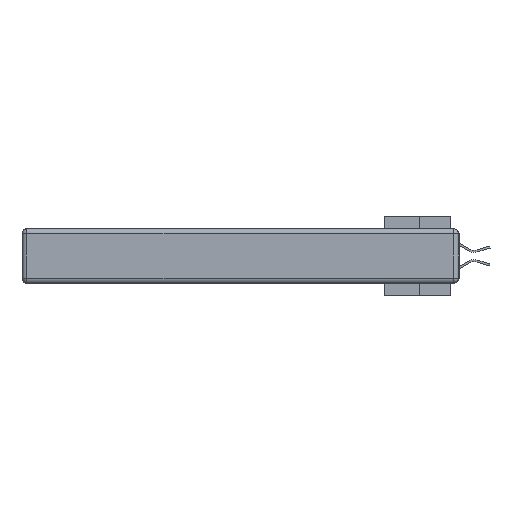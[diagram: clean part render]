
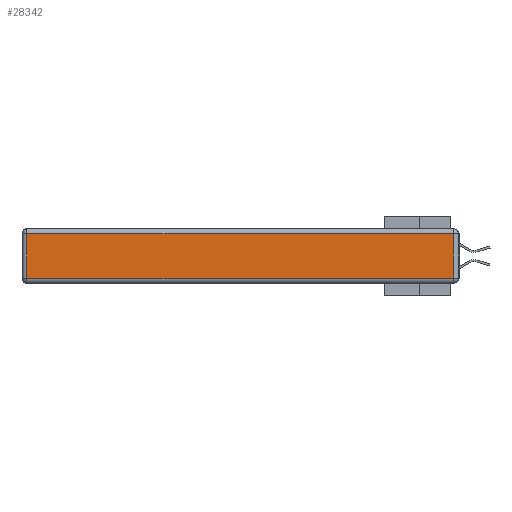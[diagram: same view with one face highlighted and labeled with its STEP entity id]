
A CAD part, left-side view. The second image highlights one B-rep face of the part: STEP entity #28342.
In plain terms, the highlighted planar face has unit normal (-1, 0, 0).
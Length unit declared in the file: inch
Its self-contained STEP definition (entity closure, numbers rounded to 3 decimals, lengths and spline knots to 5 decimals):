
#481 = CARTESIAN_POINT ( 'NONE',  ( 0., 0., -0.343 ) ) ;
#520 = CARTESIAN_POINT ( 'NONE',  ( 0., 0.03, -0.313 ) ) ;
#1318 = DIRECTION ( 'NONE',  ( 0., -1., 0. ) ) ;
#1412 = EDGE_CURVE ( 'NONE', #2188, #10132, #20508, .T. ) ;
#1446 = DIRECTION ( 'NONE',  ( 0., 0., -1. ) ) ;
#2188 = VERTEX_POINT ( 'NONE', #520 ) ;
#2374 = PLANE ( 'NONE',  #21184 ) ;
#2589 = LINE ( 'NONE', #17689, #14006 ) ;
#2668 = DIRECTION ( 'NONE',  ( -1., 0., 0. ) ) ;
#2833 = EDGE_CURVE ( 'NONE', #21985, #23923, #2589, .T. ) ;
#3038 = VECTOR ( 'NONE', #27250, 39.37008 ) ;
#4443 = LINE ( 'NONE', #10112, #27970 ) ;
#4824 = CARTESIAN_POINT ( 'NONE',  ( 0., 2.72, -0.313 ) ) ;
#4880 = DIRECTION ( 'NONE',  ( 0., 0., 1. ) ) ;
#5219 = EDGE_CURVE ( 'NONE', #10132, #21985, #16275, .T. ) ;
#5588 = VECTOR ( 'NONE', #26904, 39.37008 ) ;
#5892 = ORIENTED_EDGE ( 'NONE', *, *, #22180, .T. ) ;
#10112 = CARTESIAN_POINT ( 'NONE',  ( 0., 0., -0.313 ) ) ;
#10132 = VERTEX_POINT ( 'NONE', #18668 ) ;
#11481 = EDGE_LOOP ( 'NONE', ( #5892, #21379, #22857, #13944 ) ) ;
#13944 = ORIENTED_EDGE ( 'NONE', *, *, #2833, .T. ) ;
#14006 = VECTOR ( 'NONE', #1446, 39.37008 ) ;
#15081 = FACE_OUTER_BOUND ( 'NONE', #11481, .T. ) ;
#16275 = LINE ( 'NONE', #20440, #5588 ) ;
#17689 = CARTESIAN_POINT ( 'NONE',  ( 0., 2.72, -0.343 ) ) ;
#18668 = CARTESIAN_POINT ( 'NONE',  ( 0., 0.03, -0.03 ) ) ;
#20406 = CARTESIAN_POINT ( 'NONE',  ( 0., 0.03, -0.343 ) ) ;
#20440 = CARTESIAN_POINT ( 'NONE',  ( 0., 2.75, -0.03 ) ) ;
#20508 = LINE ( 'NONE', #20406, #3038 ) ;
#21184 = AXIS2_PLACEMENT_3D ( 'NONE', #481, #2668, #4880 ) ;
#21379 = ORIENTED_EDGE ( 'NONE', *, *, #1412, .T. ) ;
#21456 = CARTESIAN_POINT ( 'NONE',  ( 0., 2.72, -0.03 ) ) ;
#21985 = VERTEX_POINT ( 'NONE', #21456 ) ;
#22180 = EDGE_CURVE ( 'NONE', #23923, #2188, #4443, .T. ) ;
#22857 = ORIENTED_EDGE ( 'NONE', *, *, #5219, .T. ) ;
#23923 = VERTEX_POINT ( 'NONE', #4824 ) ;
#26904 = DIRECTION ( 'NONE',  ( 0., 1., 0. ) ) ;
#27250 = DIRECTION ( 'NONE',  ( 0., 0., 1. ) ) ;
#27970 = VECTOR ( 'NONE', #1318, 39.37008 ) ;
#28342 = ADVANCED_FACE ( 'NONE', ( #15081 ), #2374, .T. ) ;
